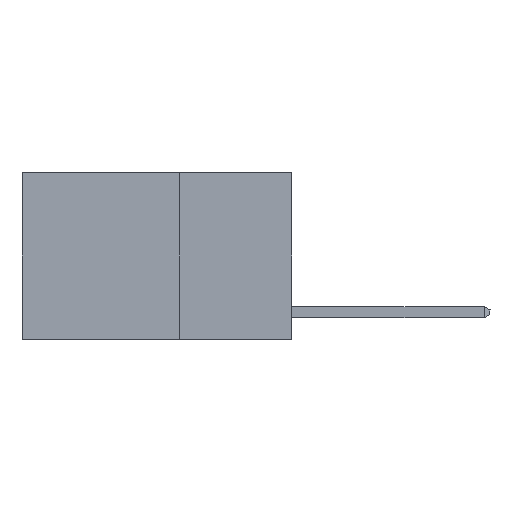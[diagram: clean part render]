
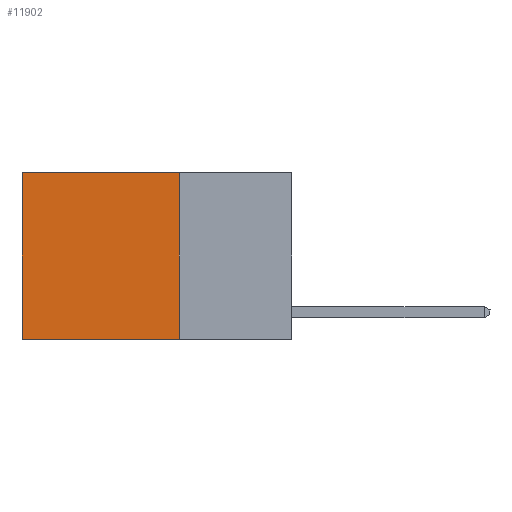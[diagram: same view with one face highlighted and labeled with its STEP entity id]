
A CAD part, left-side view. The second image highlights one B-rep face of the part: STEP entity #11902.
In plain terms, the highlighted planar face has unit normal (-1, 0, 0).
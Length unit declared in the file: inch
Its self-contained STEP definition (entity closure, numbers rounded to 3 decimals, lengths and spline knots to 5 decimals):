
#89 = CARTESIAN_POINT ( 'NONE',  ( 0.2625, 0.6, -0.37 ) ) ;
#888 = VERTEX_POINT ( 'NONE', #89 ) ;
#981 = EDGE_CURVE ( 'NONE', #25114, #29505, #24759, .T. ) ;
#2244 = CARTESIAN_POINT ( 'NONE',  ( 0.2625, 0.25, 0. ) ) ;
#2512 = DIRECTION ( 'NONE',  ( 0., 0., -1. ) ) ;
#4337 = ORIENTED_EDGE ( 'NONE', *, *, #9610, .T. ) ;
#4370 = CARTESIAN_POINT ( 'NONE',  ( 0.2625, 0.25, 0. ) ) ;
#6939 = VECTOR ( 'NONE', #25250, 39.37008 ) ;
#8097 = VECTOR ( 'NONE', #11162, 39.37008 ) ;
#9243 = CARTESIAN_POINT ( 'NONE',  ( 0.2625, 0.6, 0. ) ) ;
#9610 = EDGE_CURVE ( 'NONE', #25114, #10858, #11203, .T. ) ;
#9736 = VECTOR ( 'NONE', #11184, 39.37008 ) ;
#10743 = CARTESIAN_POINT ( 'NONE',  ( 0.2625, 0.25, 0. ) ) ;
#10858 = VERTEX_POINT ( 'NONE', #13387 ) ;
#11162 = DIRECTION ( 'NONE',  ( 0., 1., 0. ) ) ;
#11184 = DIRECTION ( 'NONE',  ( 0., 1., 0. ) ) ;
#11203 = LINE ( 'NONE', #2244, #9736 ) ;
#11902 = ADVANCED_FACE ( 'NONE', ( #22872 ), #23368, .F. ) ;
#12020 = CARTESIAN_POINT ( 'NONE',  ( 0.2625, 0.25, 0. ) ) ;
#13017 = EDGE_CURVE ( 'NONE', #29505, #888, #18175, .T. ) ;
#13387 = CARTESIAN_POINT ( 'NONE',  ( 0.2625, 0.6, 0. ) ) ;
#16130 = EDGE_CURVE ( 'NONE', #10858, #888, #23052, .T. ) ;
#16699 = AXIS2_PLACEMENT_3D ( 'NONE', #12020, #27668, #2512 ) ;
#18175 = LINE ( 'NONE', #18303, #8097 ) ;
#18303 = CARTESIAN_POINT ( 'NONE',  ( 0.2625, 0.25, -0.37 ) ) ;
#20319 = EDGE_LOOP ( 'NONE', ( #26696, #27684, #23929, #4337 ) ) ;
#22872 = FACE_OUTER_BOUND ( 'NONE', #20319, .T. ) ;
#23052 = LINE ( 'NONE', #9243, #6939 ) ;
#23368 = PLANE ( 'NONE',  #16699 ) ;
#23929 = ORIENTED_EDGE ( 'NONE', *, *, #981, .F. ) ;
#24759 = LINE ( 'NONE', #10743, #25461 ) ;
#25114 = VERTEX_POINT ( 'NONE', #4370 ) ;
#25250 = DIRECTION ( 'NONE',  ( 0., 0., -1. ) ) ;
#25461 = VECTOR ( 'NONE', #28781, 39.37008 ) ;
#26087 = CARTESIAN_POINT ( 'NONE',  ( 0.2625, 0.25, -0.37 ) ) ;
#26696 = ORIENTED_EDGE ( 'NONE', *, *, #16130, .T. ) ;
#27668 = DIRECTION ( 'NONE',  ( 1., 0., 0. ) ) ;
#27684 = ORIENTED_EDGE ( 'NONE', *, *, #13017, .F. ) ;
#28781 = DIRECTION ( 'NONE',  ( 0., 0., -1. ) ) ;
#29505 = VERTEX_POINT ( 'NONE', #26087 ) ;
